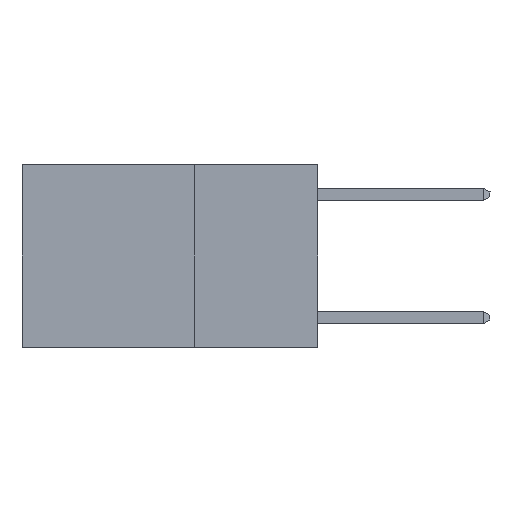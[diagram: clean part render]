
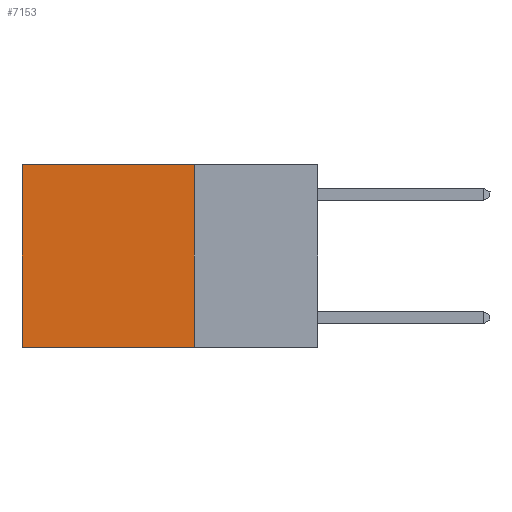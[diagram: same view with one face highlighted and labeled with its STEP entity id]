
A CAD part, left-side view. The second image highlights one B-rep face of the part: STEP entity #7153.
In plain terms, the highlighted planar face has unit normal (-1, 0, 0).
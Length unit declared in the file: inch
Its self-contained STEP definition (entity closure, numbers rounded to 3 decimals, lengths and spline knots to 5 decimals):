
#690 = CARTESIAN_POINT ( 'NONE',  ( 0.2625, 0.6, -0.37 ) ) ;
#858 = EDGE_CURVE ( 'NONE', #4770, #1782, #7259, .T. ) ;
#1632 = VECTOR ( 'NONE', #6778, 39.37008 ) ;
#1640 = LINE ( 'NONE', #7968, #1632 ) ;
#1782 = VERTEX_POINT ( 'NONE', #6868 ) ;
#2266 = FACE_OUTER_BOUND ( 'NONE', #7675, .T. ) ;
#3058 = AXIS2_PLACEMENT_3D ( 'NONE', #3521, #3389, #3388 ) ;
#3209 = LINE ( 'NONE', #7771, #3220 ) ;
#3220 = VECTOR ( 'NONE', #7765, 39.37008 ) ;
#3388 = DIRECTION ( 'NONE',  ( 0., 0., -1. ) ) ;
#3389 = DIRECTION ( 'NONE',  ( 1., 0., 0. ) ) ;
#3506 = PLANE ( 'NONE',  #3058 ) ;
#3521 = CARTESIAN_POINT ( 'NONE',  ( 0.2625, 0.25, 0. ) ) ;
#3651 = CARTESIAN_POINT ( 'NONE',  ( 0.2625, 0.6, 0. ) ) ;
#3687 = EDGE_CURVE ( 'NONE', #1782, #5762, #1640, .T. ) ;
#3736 = DIRECTION ( 'NONE',  ( 0., 1., 0. ) ) ;
#3794 = CARTESIAN_POINT ( 'NONE',  ( 0.2625, 0.25, 0. ) ) ;
#4390 = VERTEX_POINT ( 'NONE', #3651 ) ;
#4770 = VERTEX_POINT ( 'NONE', #7083 ) ;
#5164 = DIRECTION ( 'NONE',  ( 0., 0., -1. ) ) ;
#5166 = EDGE_CURVE ( 'NONE', #4770, #4390, #5796, .T. ) ;
#5762 = VERTEX_POINT ( 'NONE', #690 ) ;
#5771 = VECTOR ( 'NONE', #3736, 39.37008 ) ;
#5796 = LINE ( 'NONE', #3794, #5771 ) ;
#6591 = EDGE_CURVE ( 'NONE', #4390, #5762, #3209, .T. ) ;
#6778 = DIRECTION ( 'NONE',  ( 0., 1., 0. ) ) ;
#6868 = CARTESIAN_POINT ( 'NONE',  ( 0.2625, 0.25, -0.37 ) ) ;
#6930 = CARTESIAN_POINT ( 'NONE',  ( 0.2625, 0.25, 0. ) ) ;
#7083 = CARTESIAN_POINT ( 'NONE',  ( 0.2625, 0.25, 0. ) ) ;
#7153 = ADVANCED_FACE ( 'NONE', ( #2266 ), #3506, .F. ) ;
#7229 = VECTOR ( 'NONE', #5164, 39.37008 ) ;
#7259 = LINE ( 'NONE', #6930, #7229 ) ;
#7675 = EDGE_LOOP ( 'NONE', ( #7876, #7881, #7921, #8142 ) ) ;
#7765 = DIRECTION ( 'NONE',  ( 0., 0., -1. ) ) ;
#7771 = CARTESIAN_POINT ( 'NONE',  ( 0.2625, 0.6, 0. ) ) ;
#7876 = ORIENTED_EDGE ( 'NONE', *, *, #6591, .T. ) ;
#7881 = ORIENTED_EDGE ( 'NONE', *, *, #3687, .F. ) ;
#7921 = ORIENTED_EDGE ( 'NONE', *, *, #858, .F. ) ;
#7968 = CARTESIAN_POINT ( 'NONE',  ( 0.2625, 0.25, -0.37 ) ) ;
#8142 = ORIENTED_EDGE ( 'NONE', *, *, #5166, .T. ) ;
